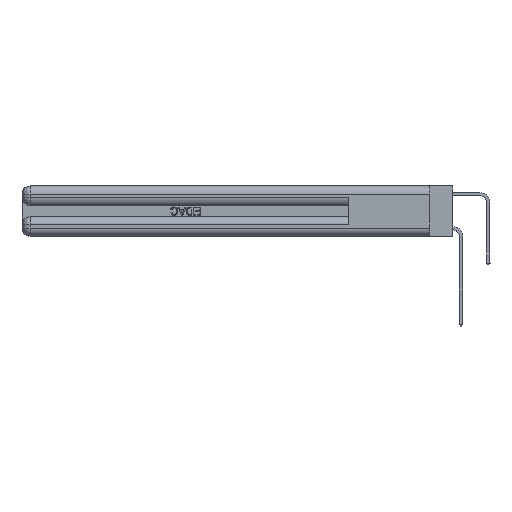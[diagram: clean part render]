
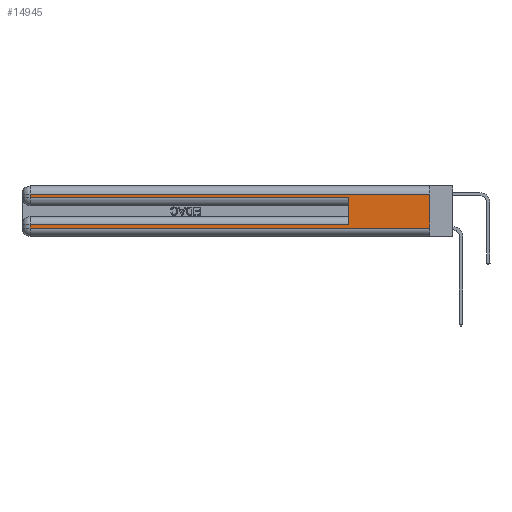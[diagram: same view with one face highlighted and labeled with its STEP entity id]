
A CAD part, left-side view. The second image highlights one B-rep face of the part: STEP entity #14945.
In plain terms, the highlighted planar face has unit normal (-1, 0, 0).
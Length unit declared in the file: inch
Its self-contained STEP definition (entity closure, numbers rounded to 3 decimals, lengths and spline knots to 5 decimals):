
#1126 = EDGE_CURVE ( 'NONE', #8007, #23616, #15296, .T. ) ;
#1196 = EDGE_CURVE ( 'NONE', #26446, #18427, #30579, .T. ) ;
#1238 = ORIENTED_EDGE ( 'NONE', *, *, #1126, .T. ) ;
#1815 = CARTESIAN_POINT ( 'NONE',  ( 0., 0., 0.285 ) ) ;
#2940 = PLANE ( 'NONE',  #16517 ) ;
#3960 = ORIENTED_EDGE ( 'NONE', *, *, #20496, .T. ) ;
#6533 = EDGE_CURVE ( 'NONE', #23616, #7594, #20751, .T. ) ;
#6730 = VECTOR ( 'NONE', #16007, 39.37008 ) ;
#7594 = VERTEX_POINT ( 'NONE', #16644 ) ;
#7864 = CARTESIAN_POINT ( 'NONE',  ( 0., 2.94, 0.085 ) ) ;
#8007 = VERTEX_POINT ( 'NONE', #24508 ) ;
#8314 = FACE_OUTER_BOUND ( 'NONE', #15806, .T. ) ;
#8856 = CARTESIAN_POINT ( 'NONE',  ( 0., 0., 0.37 ) ) ;
#9571 = CARTESIAN_POINT ( 'NONE',  ( 0., 2.94, 0.31 ) ) ;
#9979 = LINE ( 'NONE', #21416, #6730 ) ;
#10224 = LINE ( 'NONE', #1815, #18747 ) ;
#10492 = CARTESIAN_POINT ( 'NONE',  ( 0., 0.6, 0.285 ) ) ;
#10974 = ORIENTED_EDGE ( 'NONE', *, *, #26353, .F. ) ;
#11526 = CARTESIAN_POINT ( 'NONE',  ( 0., 0.6, 0.085 ) ) ;
#13134 = CARTESIAN_POINT ( 'NONE',  ( 0., 0., 0.31 ) ) ;
#13736 = EDGE_CURVE ( 'NONE', #7594, #32161, #10224, .T. ) ;
#14030 = CARTESIAN_POINT ( 'NONE',  ( 0., 0., 0.085 ) ) ;
#14945 = ADVANCED_FACE ( 'NONE', ( #8314 ), #2940, .F. ) ;
#15296 = LINE ( 'NONE', #13134, #26213 ) ;
#15599 = ORIENTED_EDGE ( 'NONE', *, *, #6533, .T. ) ;
#15806 = EDGE_LOOP ( 'NONE', ( #10974, #1238, #15599, #35253, #16417, #27848, #3960, #29993 ) ) ;
#16007 = DIRECTION ( 'NONE',  ( 0., 0., -1. ) ) ;
#16417 = ORIENTED_EDGE ( 'NONE', *, *, #24756, .F. ) ;
#16517 = AXIS2_PLACEMENT_3D ( 'NONE', #8856, #19256, #32943 ) ;
#16644 = CARTESIAN_POINT ( 'NONE',  ( 0., 2.94, 0.285 ) ) ;
#17504 = VECTOR ( 'NONE', #17515, 39.37008 ) ;
#17515 = DIRECTION ( 'NONE',  ( 0., 0., -1. ) ) ;
#17817 = VECTOR ( 'NONE', #23600, 39.37008 ) ;
#18427 = VERTEX_POINT ( 'NONE', #7864 ) ;
#18621 = LINE ( 'NONE', #32655, #26560 ) ;
#18747 = VECTOR ( 'NONE', #31971, 39.37008 ) ;
#18879 = DIRECTION ( 'NONE',  ( 0., 1., 0. ) ) ;
#19256 = DIRECTION ( 'NONE',  ( 1., 0., 0. ) ) ;
#20376 = VERTEX_POINT ( 'NONE', #27589 ) ;
#20496 = EDGE_CURVE ( 'NONE', #18427, #20376, #25770, .T. ) ;
#20751 = LINE ( 'NONE', #31199, #17504 ) ;
#21416 = CARTESIAN_POINT ( 'NONE',  ( 0., 0., 0.37 ) ) ;
#21507 = DIRECTION ( 'NONE',  ( 0., -1., 0. ) ) ;
#22184 = VERTEX_POINT ( 'NONE', #26065 ) ;
#22728 = EDGE_CURVE ( 'NONE', #20376, #22184, #18621, .T. ) ;
#23600 = DIRECTION ( 'NONE',  ( 0., 0., -1. ) ) ;
#23616 = VERTEX_POINT ( 'NONE', #9571 ) ;
#24508 = CARTESIAN_POINT ( 'NONE',  ( 0., 0., 0.31 ) ) ;
#24756 = EDGE_CURVE ( 'NONE', #26446, #32161, #31165, .T. ) ;
#25770 = LINE ( 'NONE', #29001, #17817 ) ;
#26065 = CARTESIAN_POINT ( 'NONE',  ( 0., 0., 0.06 ) ) ;
#26213 = VECTOR ( 'NONE', #32208, 39.37008 ) ;
#26353 = EDGE_CURVE ( 'NONE', #8007, #22184, #9979, .T. ) ;
#26446 = VERTEX_POINT ( 'NONE', #11526 ) ;
#26560 = VECTOR ( 'NONE', #21507, 39.37008 ) ;
#27589 = CARTESIAN_POINT ( 'NONE',  ( 0., 2.94, 0.06 ) ) ;
#27848 = ORIENTED_EDGE ( 'NONE', *, *, #1196, .T. ) ;
#29001 = CARTESIAN_POINT ( 'NONE',  ( 0., 2.94, 0.37 ) ) ;
#29993 = ORIENTED_EDGE ( 'NONE', *, *, #22728, .T. ) ;
#30236 = VECTOR ( 'NONE', #18879, 39.37008 ) ;
#30579 = LINE ( 'NONE', #14030, #30236 ) ;
#31165 = LINE ( 'NONE', #33866, #31263 ) ;
#31199 = CARTESIAN_POINT ( 'NONE',  ( 0., 2.94, 0.37 ) ) ;
#31263 = VECTOR ( 'NONE', #34224, 39.37008 ) ;
#31971 = DIRECTION ( 'NONE',  ( 0., -1., 0. ) ) ;
#32161 = VERTEX_POINT ( 'NONE', #10492 ) ;
#32208 = DIRECTION ( 'NONE',  ( 0., 1., 0. ) ) ;
#32655 = CARTESIAN_POINT ( 'NONE',  ( 0., 0., 0.06 ) ) ;
#32943 = DIRECTION ( 'NONE',  ( 0., 0., -1. ) ) ;
#33866 = CARTESIAN_POINT ( 'NONE',  ( 0., 0.6, 0.145 ) ) ;
#34224 = DIRECTION ( 'NONE',  ( 0., 0., 1. ) ) ;
#35253 = ORIENTED_EDGE ( 'NONE', *, *, #13736, .T. ) ;
